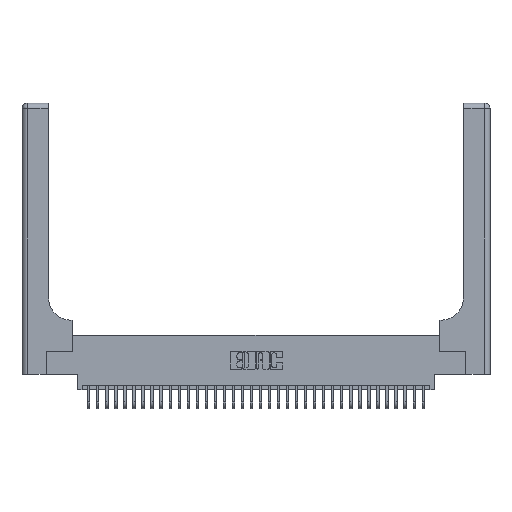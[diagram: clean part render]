
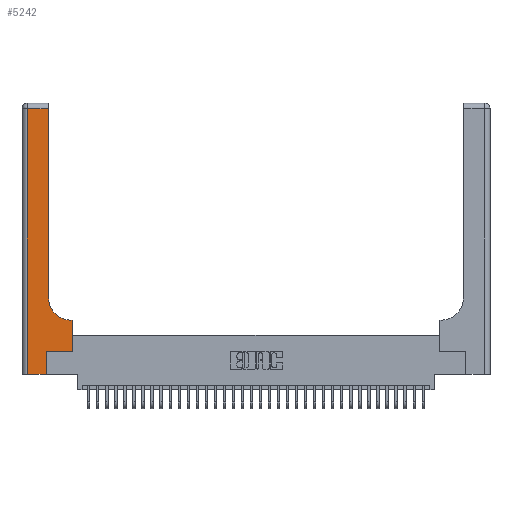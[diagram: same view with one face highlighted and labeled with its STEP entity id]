
A CAD part, top view. The second image highlights one B-rep face of the part: STEP entity #5242.
In plain terms, the highlighted planar face has unit normal (0, 0, 1).
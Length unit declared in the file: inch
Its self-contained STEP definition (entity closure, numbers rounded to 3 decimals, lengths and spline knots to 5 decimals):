
#154 = EDGE_CURVE ( 'NONE', #4546, #34001, #33999, .T. ) ;
#494 = ORIENTED_EDGE ( 'NONE', *, *, #1975, .T. ) ;
#553 = VERTEX_POINT ( 'NONE', #25625 ) ;
#1022 = LINE ( 'NONE', #23171, #16391 ) ;
#1308 = LINE ( 'NONE', #19890, #7152 ) ;
#1746 = EDGE_CURVE ( 'NONE', #34001, #6519, #18040, .T. ) ;
#1774 = DIRECTION ( 'NONE',  ( 1., 0., 0. ) ) ;
#1975 = EDGE_CURVE ( 'NONE', #553, #4546, #34753, .T. ) ;
#1996 = VECTOR ( 'NONE', #13016, 39.37008 ) ;
#2249 = LINE ( 'NONE', #2875, #31546 ) ;
#2875 = CARTESIAN_POINT ( 'NONE',  ( 0.06, 3., 0.37 ) ) ;
#3501 = VECTOR ( 'NONE', #28556, 39.37008 ) ;
#3567 = AXIS2_PLACEMENT_3D ( 'NONE', #22349, #19297, #5308 ) ;
#4546 = VERTEX_POINT ( 'NONE', #34009 ) ;
#5200 = DIRECTION ( 'NONE',  ( 1., 0., 0. ) ) ;
#5242 = ADVANCED_FACE ( 'NONE', ( #17400 ), #24974, .F. ) ;
#5308 = DIRECTION ( 'NONE',  ( -1., 0., 0. ) ) ;
#5823 = DIRECTION ( 'NONE',  ( 0., 0., -1. ) ) ;
#6519 = VERTEX_POINT ( 'NONE', #24388 ) ;
#6572 = EDGE_CURVE ( 'NONE', #6519, #23366, #2249, .T. ) ;
#6587 = ORIENTED_EDGE ( 'NONE', *, *, #26244, .T. ) ;
#7152 = VECTOR ( 'NONE', #34614, 39.37008 ) ;
#7412 = ORIENTED_EDGE ( 'NONE', *, *, #14413, .T. ) ;
#8024 = CARTESIAN_POINT ( 'NONE',  ( 0.06, 0., 0.37 ) ) ;
#8316 = EDGE_CURVE ( 'NONE', #32989, #22950, #32346, .T. ) ;
#10575 = ORIENTED_EDGE ( 'NONE', *, *, #154, .T. ) ;
#11797 = ORIENTED_EDGE ( 'NONE', *, *, #34652, .T. ) ;
#11984 = VERTEX_POINT ( 'NONE', #30717 ) ;
#12765 = DIRECTION ( 'NONE',  ( -1., 0., 0. ) ) ;
#13016 = DIRECTION ( 'NONE',  ( 0., 1., 0. ) ) ;
#14413 = EDGE_CURVE ( 'NONE', #11984, #553, #1022, .T. ) ;
#16274 = CARTESIAN_POINT ( 'NONE',  ( 0.269, 0.25, 0.37 ) ) ;
#16285 = CARTESIAN_POINT ( 'NONE',  ( 0.2915, 3., 0.37 ) ) ;
#16391 = VECTOR ( 'NONE', #33468, 39.37008 ) ;
#16739 = CARTESIAN_POINT ( 'NONE',  ( 0.2915, 2.94, 0.37 ) ) ;
#17078 = CARTESIAN_POINT ( 'NONE',  ( 0.5585, 0.25, 0.37 ) ) ;
#17400 = FACE_OUTER_BOUND ( 'NONE', #35468, .T. ) ;
#18040 = LINE ( 'NONE', #32150, #19899 ) ;
#19297 = DIRECTION ( 'NONE',  ( 0., 0., -1. ) ) ;
#19890 = CARTESIAN_POINT ( 'NONE',  ( 0.5585, 0.25, 0.37 ) ) ;
#19899 = VECTOR ( 'NONE', #12765, 39.37008 ) ;
#20094 = CARTESIAN_POINT ( 'NONE',  ( 0.269, 0., 0.37 ) ) ;
#21923 = VERTEX_POINT ( 'NONE', #17078 ) ;
#22331 = ORIENTED_EDGE ( 'NONE', *, *, #6572, .T. ) ;
#22349 = CARTESIAN_POINT ( 'NONE',  ( 0., 3., 0.37 ) ) ;
#22870 = ORIENTED_EDGE ( 'NONE', *, *, #1746, .T. ) ;
#22872 = LINE ( 'NONE', #16274, #26015 ) ;
#22950 = VERTEX_POINT ( 'NONE', #30359 ) ;
#23166 = ORIENTED_EDGE ( 'NONE', *, *, #8316, .T. ) ;
#23171 = CARTESIAN_POINT ( 'NONE',  ( 0.2915, 0.6, 0.37 ) ) ;
#23366 = VERTEX_POINT ( 'NONE', #8024 ) ;
#24388 = CARTESIAN_POINT ( 'NONE',  ( 0.06, 2.94, 0.37 ) ) ;
#24974 = PLANE ( 'NONE',  #3567 ) ;
#25264 = EDGE_CURVE ( 'NONE', #21923, #11984, #1308, .T. ) ;
#25625 = CARTESIAN_POINT ( 'NONE',  ( 0.5415, 0.6, 0.37 ) ) ;
#25872 = CARTESIAN_POINT ( 'NONE',  ( 0.5415, 0.85, 0.37 ) ) ;
#25991 = DIRECTION ( 'NONE',  ( 1., 0., 0. ) ) ;
#26015 = VECTOR ( 'NONE', #1774, 39.37008 ) ;
#26244 = EDGE_CURVE ( 'NONE', #22950, #21923, #22872, .T. ) ;
#26764 = DIRECTION ( 'NONE',  ( 0., -1., 0. ) ) ;
#26923 = AXIS2_PLACEMENT_3D ( 'NONE', #25872, #5823, #25991 ) ;
#28064 = ORIENTED_EDGE ( 'NONE', *, *, #25264, .T. ) ;
#28556 = DIRECTION ( 'NONE',  ( 0., 1., 0. ) ) ;
#28651 = CARTESIAN_POINT ( 'NONE',  ( 0.269, 0., 0.37 ) ) ;
#28783 = CARTESIAN_POINT ( 'NONE',  ( 0., 0., 0.37 ) ) ;
#30359 = CARTESIAN_POINT ( 'NONE',  ( 0.269, 0.25, 0.37 ) ) ;
#30717 = CARTESIAN_POINT ( 'NONE',  ( 0.5585, 0.6, 0.37 ) ) ;
#31546 = VECTOR ( 'NONE', #26764, 39.37008 ) ;
#31604 = LINE ( 'NONE', #28783, #32951 ) ;
#32150 = CARTESIAN_POINT ( 'NONE',  ( 0., 2.94, 0.37 ) ) ;
#32346 = LINE ( 'NONE', #20094, #3501 ) ;
#32951 = VECTOR ( 'NONE', #5200, 39.37008 ) ;
#32989 = VERTEX_POINT ( 'NONE', #28651 ) ;
#33468 = DIRECTION ( 'NONE',  ( -1., 0., 0. ) ) ;
#33999 = LINE ( 'NONE', #16285, #1996 ) ;
#34001 = VERTEX_POINT ( 'NONE', #16739 ) ;
#34009 = CARTESIAN_POINT ( 'NONE',  ( 0.2915, 0.85, 0.37 ) ) ;
#34614 = DIRECTION ( 'NONE',  ( 0., 1., 0. ) ) ;
#34652 = EDGE_CURVE ( 'NONE', #23366, #32989, #31604, .T. ) ;
#34753 = CIRCLE ( 'NONE', #26923, 0.25 ) ;
#35468 = EDGE_LOOP ( 'NONE', ( #10575, #22870, #22331, #11797, #23166, #6587, #28064, #7412, #494 ) ) ;
